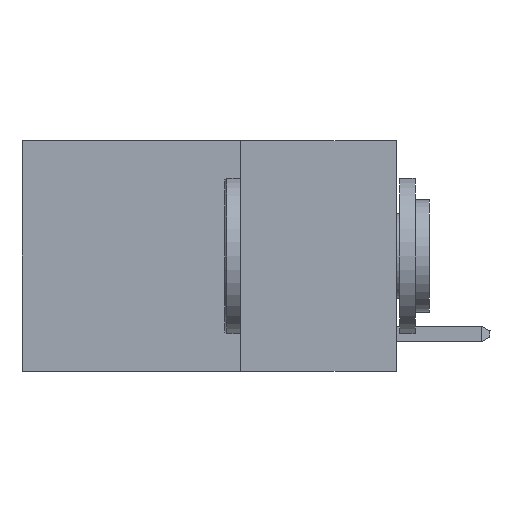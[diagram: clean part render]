
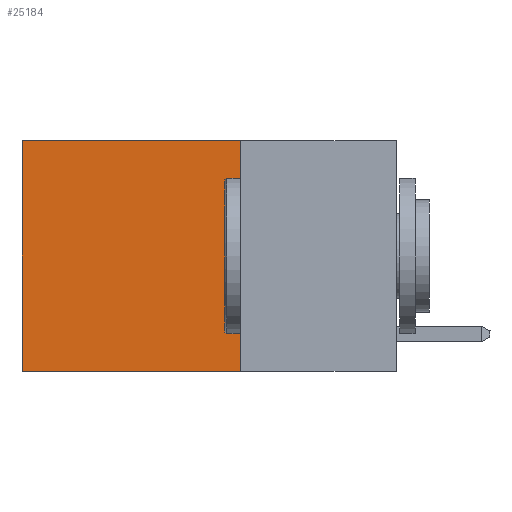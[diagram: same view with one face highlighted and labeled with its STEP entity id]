
A CAD part, left-side view. The second image highlights one B-rep face of the part: STEP entity #25184.
In plain terms, the highlighted planar face has unit normal (-1, 0, 0).
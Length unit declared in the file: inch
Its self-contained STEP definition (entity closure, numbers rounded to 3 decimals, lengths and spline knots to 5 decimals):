
#570 = CARTESIAN_POINT ( 'NONE',  ( 0.2625, 0.6, 0. ) ) ;
#2222 = PLANE ( 'NONE',  #4613 ) ;
#2428 = DIRECTION ( 'NONE',  ( 0., 0., -1. ) ) ;
#2744 = EDGE_CURVE ( 'NONE', #16905, #17280, #23861, .T. ) ;
#2970 = CARTESIAN_POINT ( 'NONE',  ( 0.2625, 0.25, 0. ) ) ;
#3633 = VERTEX_POINT ( 'NONE', #20731 ) ;
#3662 = LINE ( 'NONE', #9431, #13740 ) ;
#4613 = AXIS2_PLACEMENT_3D ( 'NONE', #12027, #6386, #15810 ) ;
#5088 = EDGE_CURVE ( 'NONE', #17280, #17881, #3662, .T. ) ;
#5740 = FACE_OUTER_BOUND ( 'NONE', #17857, .T. ) ;
#6386 = DIRECTION ( 'NONE',  ( 1., 0., 0. ) ) ;
#8417 = ORIENTED_EDGE ( 'NONE', *, *, #5088, .T. ) ;
#9431 = CARTESIAN_POINT ( 'NONE',  ( 0.2625, 0.6, 0. ) ) ;
#10390 = VECTOR ( 'NONE', #21404, 39.37008 ) ;
#11264 = DIRECTION ( 'NONE',  ( 0., 1., 0. ) ) ;
#11655 = VECTOR ( 'NONE', #19465, 39.37008 ) ;
#11668 = ORIENTED_EDGE ( 'NONE', *, *, #23648, .F. ) ;
#12027 = CARTESIAN_POINT ( 'NONE',  ( 0.2625, 0.25, 0. ) ) ;
#13141 = CARTESIAN_POINT ( 'NONE',  ( 0.2625, 0.6, -0.37 ) ) ;
#13740 = VECTOR ( 'NONE', #2428, 39.37008 ) ;
#15537 = CARTESIAN_POINT ( 'NONE',  ( 0.2625, 0.25, -0.37 ) ) ;
#15810 = DIRECTION ( 'NONE',  ( 0., 0., -1. ) ) ;
#16905 = VERTEX_POINT ( 'NONE', #2970 ) ;
#17133 = LINE ( 'NONE', #15537, #10390 ) ;
#17280 = VERTEX_POINT ( 'NONE', #570 ) ;
#17555 = EDGE_CURVE ( 'NONE', #16905, #3633, #20577, .T. ) ;
#17857 = EDGE_LOOP ( 'NONE', ( #8417, #11668, #21069, #18743 ) ) ;
#17881 = VERTEX_POINT ( 'NONE', #13141 ) ;
#18743 = ORIENTED_EDGE ( 'NONE', *, *, #2744, .T. ) ;
#19009 = VECTOR ( 'NONE', #11264, 39.37008 ) ;
#19465 = DIRECTION ( 'NONE',  ( 0., 0., -1. ) ) ;
#20577 = LINE ( 'NONE', #21510, #11655 ) ;
#20731 = CARTESIAN_POINT ( 'NONE',  ( 0.2625, 0.25, -0.37 ) ) ;
#21069 = ORIENTED_EDGE ( 'NONE', *, *, #17555, .F. ) ;
#21404 = DIRECTION ( 'NONE',  ( 0., 1., 0. ) ) ;
#21510 = CARTESIAN_POINT ( 'NONE',  ( 0.2625, 0.25, 0. ) ) ;
#23140 = CARTESIAN_POINT ( 'NONE',  ( 0.2625, 0.25, 0. ) ) ;
#23648 = EDGE_CURVE ( 'NONE', #3633, #17881, #17133, .T. ) ;
#23861 = LINE ( 'NONE', #23140, #19009 ) ;
#25184 = ADVANCED_FACE ( 'NONE', ( #5740 ), #2222, .F. ) ;
